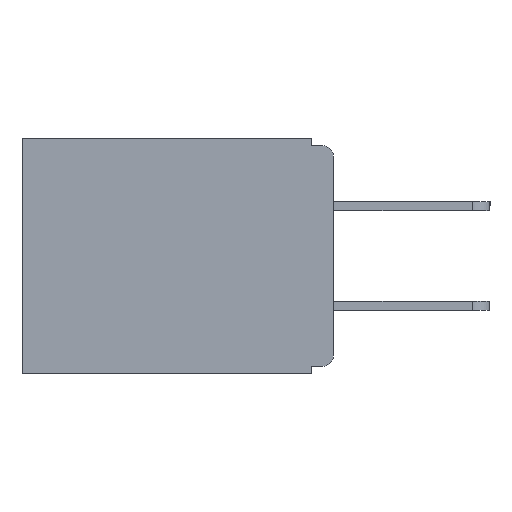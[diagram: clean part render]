
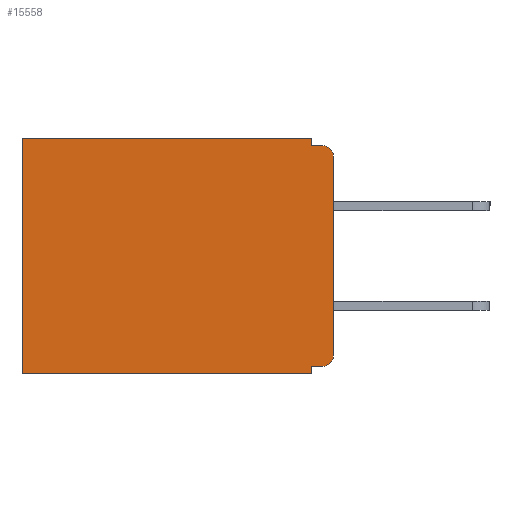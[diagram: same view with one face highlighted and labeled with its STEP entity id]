
A CAD part, left-side view. The second image highlights one B-rep face of the part: STEP entity #15558.
In plain terms, the highlighted planar face has unit normal (-1, 0, 0).
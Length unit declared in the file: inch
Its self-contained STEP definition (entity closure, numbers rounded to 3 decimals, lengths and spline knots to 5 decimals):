
#59 = ORIENTED_EDGE ( 'NONE', *, *, #10785, .F. ) ;
#350 = CARTESIAN_POINT ( 'NONE',  ( 0.3, 0.015, -0.305 ) ) ;
#941 = CARTESIAN_POINT ( 'NONE',  ( 0.3, 0.015, -0.01 ) ) ;
#1707 = CARTESIAN_POINT ( 'NONE',  ( 0.3, 0., -0.33 ) ) ;
#1841 = DIRECTION ( 'NONE',  ( 0., 0., -1. ) ) ;
#2632 = DIRECTION ( 'NONE',  ( 0., 0., -1. ) ) ;
#2852 = VERTEX_POINT ( 'NONE', #19304 ) ;
#3198 = EDGE_CURVE ( 'NONE', #22726, #15656, #14920, .T. ) ;
#3696 = VECTOR ( 'NONE', #19240, 39.37008 ) ;
#3904 = CARTESIAN_POINT ( 'NONE',  ( 0.3, 0.437, 0. ) ) ;
#3938 = CARTESIAN_POINT ( 'NONE',  ( 0.3, 0.031, -0.01 ) ) ;
#3976 = DIRECTION ( 'NONE',  ( 1., 0., 0. ) ) ;
#4325 = VECTOR ( 'NONE', #28374, 39.37008 ) ;
#4330 = LINE ( 'NONE', #5193, #15586 ) ;
#5193 = CARTESIAN_POINT ( 'NONE',  ( 0.3, 0., -0.33 ) ) ;
#5433 = LINE ( 'NONE', #19710, #16699 ) ;
#5624 = FACE_OUTER_BOUND ( 'NONE', #7736, .T. ) ;
#6061 = CARTESIAN_POINT ( 'NONE',  ( 0.3, 0.031, -0.33 ) ) ;
#6421 = ORIENTED_EDGE ( 'NONE', *, *, #13927, .F. ) ;
#6600 = VERTEX_POINT ( 'NONE', #11445 ) ;
#7060 = VERTEX_POINT ( 'NONE', #3904 ) ;
#7444 = DIRECTION ( 'NONE',  ( 0., 0., -1. ) ) ;
#7466 = DIRECTION ( 'NONE',  ( 0., 1., 0. ) ) ;
#7736 = EDGE_LOOP ( 'NONE', ( #23505, #24231, #59, #6421, #8553, #17720, #23592, #8581, #14936, #24698 ) ) ;
#8349 = CARTESIAN_POINT ( 'NONE',  ( 0.3, 0.015, -0.025 ) ) ;
#8553 = ORIENTED_EDGE ( 'NONE', *, *, #19252, .T. ) ;
#8581 = ORIENTED_EDGE ( 'NONE', *, *, #10959, .F. ) ;
#9476 = DIRECTION ( 'NONE',  ( 0., 0., -1. ) ) ;
#10573 = CARTESIAN_POINT ( 'NONE',  ( 0.3, 0.437, -0.33 ) ) ;
#10651 = DIRECTION ( 'NONE',  ( 0., 0., -1. ) ) ;
#10785 = EDGE_CURVE ( 'NONE', #18004, #25621, #15657, .T. ) ;
#10959 = EDGE_CURVE ( 'NONE', #15656, #12963, #5433, .T. ) ;
#11445 = CARTESIAN_POINT ( 'NONE',  ( 0.3, 0.437, -0.33 ) ) ;
#12044 = EDGE_CURVE ( 'NONE', #7060, #6600, #21489, .T. ) ;
#12963 = VERTEX_POINT ( 'NONE', #6061 ) ;
#13548 = LINE ( 'NONE', #16386, #18106 ) ;
#13927 = EDGE_CURVE ( 'NONE', #2852, #18004, #14183, .T. ) ;
#13996 = CARTESIAN_POINT ( 'NONE',  ( 0.3, 0., -0.305 ) ) ;
#14183 = LINE ( 'NONE', #22827, #26014 ) ;
#14214 = VECTOR ( 'NONE', #27282, 39.37008 ) ;
#14920 = LINE ( 'NONE', #27063, #14214 ) ;
#14936 = ORIENTED_EDGE ( 'NONE', *, *, #3198, .F. ) ;
#15171 = PLANE ( 'NONE',  #19625 ) ;
#15558 = ADVANCED_FACE ( 'NONE', ( #5624 ), #15171, .F. ) ;
#15586 = VECTOR ( 'NONE', #7466, 39.37008 ) ;
#15656 = VERTEX_POINT ( 'NONE', #19872 ) ;
#15657 = LINE ( 'NONE', #16988, #3696 ) ;
#16089 = DIRECTION ( 'NONE',  ( -1., 0., 0. ) ) ;
#16386 = CARTESIAN_POINT ( 'NONE',  ( 0.3, 0., -0.33 ) ) ;
#16699 = VECTOR ( 'NONE', #1841, 39.37008 ) ;
#16988 = CARTESIAN_POINT ( 'NONE',  ( 0.3, 0., -0.01 ) ) ;
#17720 = ORIENTED_EDGE ( 'NONE', *, *, #12044, .T. ) ;
#18004 = VERTEX_POINT ( 'NONE', #3938 ) ;
#18104 = CARTESIAN_POINT ( 'NONE',  ( 0.3, 0.015, -0.32 ) ) ;
#18106 = VECTOR ( 'NONE', #7444, 39.37008 ) ;
#18671 = CARTESIAN_POINT ( 'NONE',  ( 0.3, 0., 0. ) ) ;
#19240 = DIRECTION ( 'NONE',  ( 0., -1., 0. ) ) ;
#19252 = EDGE_CURVE ( 'NONE', #2852, #7060, #25388, .T. ) ;
#19304 = CARTESIAN_POINT ( 'NONE',  ( 0.3, 0.031, 0. ) ) ;
#19581 = AXIS2_PLACEMENT_3D ( 'NONE', #8349, #23958, #10651 ) ;
#19625 = AXIS2_PLACEMENT_3D ( 'NONE', #1707, #3976, #19684 ) ;
#19684 = DIRECTION ( 'NONE',  ( 0., 0., -1. ) ) ;
#19710 = CARTESIAN_POINT ( 'NONE',  ( 0.3, 0.031, -0.33 ) ) ;
#19767 = EDGE_CURVE ( 'NONE', #28191, #26167, #13548, .T. ) ;
#19872 = CARTESIAN_POINT ( 'NONE',  ( 0.3, 0.031, -0.32 ) ) ;
#20213 = VECTOR ( 'NONE', #25235, 39.37008 ) ;
#21146 = CARTESIAN_POINT ( 'NONE',  ( 0.3, 0., -0.025 ) ) ;
#21489 = LINE ( 'NONE', #10573, #4325 ) ;
#22726 = VERTEX_POINT ( 'NONE', #18104 ) ;
#22827 = CARTESIAN_POINT ( 'NONE',  ( 0.3, 0.031, 0. ) ) ;
#22875 = EDGE_CURVE ( 'NONE', #12963, #6600, #4330, .T. ) ;
#23271 = EDGE_CURVE ( 'NONE', #22726, #26167, #25606, .T. ) ;
#23505 = ORIENTED_EDGE ( 'NONE', *, *, #19767, .F. ) ;
#23592 = ORIENTED_EDGE ( 'NONE', *, *, #22875, .F. ) ;
#23958 = DIRECTION ( 'NONE',  ( -1., 0., 0. ) ) ;
#24231 = ORIENTED_EDGE ( 'NONE', *, *, #27738, .T. ) ;
#24412 = CIRCLE ( 'NONE', #19581, 0.015 ) ;
#24698 = ORIENTED_EDGE ( 'NONE', *, *, #23271, .T. ) ;
#25235 = DIRECTION ( 'NONE',  ( 0., 1., 0. ) ) ;
#25388 = LINE ( 'NONE', #18671, #20213 ) ;
#25606 = CIRCLE ( 'NONE', #26905, 0.015 ) ;
#25621 = VERTEX_POINT ( 'NONE', #941 ) ;
#26014 = VECTOR ( 'NONE', #9476, 39.37008 ) ;
#26167 = VERTEX_POINT ( 'NONE', #13996 ) ;
#26905 = AXIS2_PLACEMENT_3D ( 'NONE', #350, #16089, #2632 ) ;
#27063 = CARTESIAN_POINT ( 'NONE',  ( 0.3, 0., -0.32 ) ) ;
#27282 = DIRECTION ( 'NONE',  ( 0., 1., 0. ) ) ;
#27738 = EDGE_CURVE ( 'NONE', #28191, #25621, #24412, .T. ) ;
#28191 = VERTEX_POINT ( 'NONE', #21146 ) ;
#28374 = DIRECTION ( 'NONE',  ( 0., 0., -1. ) ) ;
